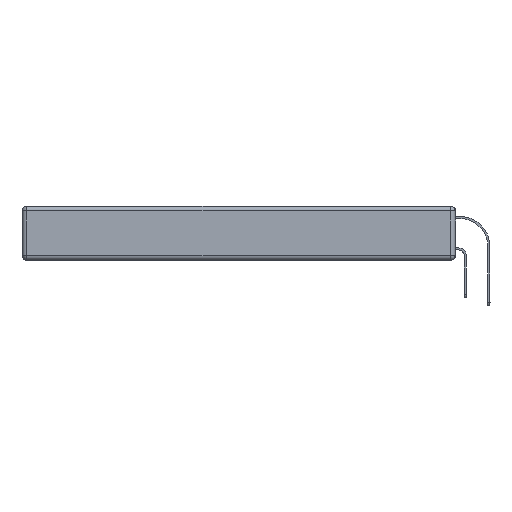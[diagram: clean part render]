
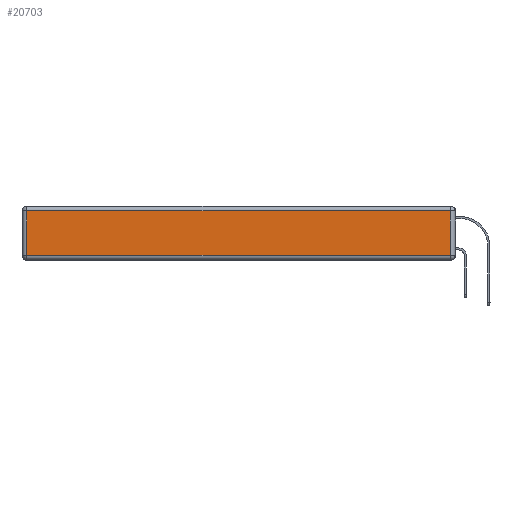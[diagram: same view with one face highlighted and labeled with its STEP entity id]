
A CAD part, left-side view. The second image highlights one B-rep face of the part: STEP entity #20703.
In plain terms, the highlighted planar face has unit normal (-1, 0, 0).
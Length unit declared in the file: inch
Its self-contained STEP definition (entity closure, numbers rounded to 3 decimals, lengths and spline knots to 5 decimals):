
#578 = VERTEX_POINT ( 'NONE', #16079 ) ;
#749 = EDGE_CURVE ( 'NONE', #12859, #14112, #18726, .T. ) ;
#1643 = VECTOR ( 'NONE', #2387, 39.37008 ) ;
#2387 = DIRECTION ( 'NONE',  ( 0., -1., 0. ) ) ;
#2833 = DIRECTION ( 'NONE',  ( 0., 0., 1. ) ) ;
#3191 = DIRECTION ( 'NONE',  ( 0., 0., 1. ) ) ;
#3199 = VERTEX_POINT ( 'NONE', #7223 ) ;
#3409 = VECTOR ( 'NONE', #21906, 39.37008 ) ;
#3702 = EDGE_CURVE ( 'NONE', #578, #3199, #10713, .T. ) ;
#4366 = ORIENTED_EDGE ( 'NONE', *, *, #13947, .T. ) ;
#4716 = EDGE_CURVE ( 'NONE', #3199, #12859, #5184, .T. ) ;
#5184 = LINE ( 'NONE', #16341, #3409 ) ;
#5561 = ORIENTED_EDGE ( 'NONE', *, *, #4716, .T. ) ;
#7223 = CARTESIAN_POINT ( 'NONE',  ( 0., 0.03, -0.03 ) ) ;
#7793 = ORIENTED_EDGE ( 'NONE', *, *, #749, .T. ) ;
#8169 = AXIS2_PLACEMENT_3D ( 'NONE', #17513, #13875, #2833 ) ;
#10346 = FACE_OUTER_BOUND ( 'NONE', #13433, .T. ) ;
#10713 = LINE ( 'NONE', #23314, #14962 ) ;
#11607 = LINE ( 'NONE', #19000, #1643 ) ;
#12859 = VERTEX_POINT ( 'NONE', #22223 ) ;
#13433 = EDGE_LOOP ( 'NONE', ( #4366, #23909, #5561, #7793 ) ) ;
#13875 = DIRECTION ( 'NONE',  ( -1., 0., 0. ) ) ;
#13947 = EDGE_CURVE ( 'NONE', #14112, #578, #11607, .T. ) ;
#14112 = VERTEX_POINT ( 'NONE', #21745 ) ;
#14962 = VECTOR ( 'NONE', #3191, 39.37008 ) ;
#16079 = CARTESIAN_POINT ( 'NONE',  ( 0., 0.03, -0.313 ) ) ;
#16341 = CARTESIAN_POINT ( 'NONE',  ( 0., 2.75, -0.03 ) ) ;
#17179 = VECTOR ( 'NONE', #22000, 39.37008 ) ;
#17513 = CARTESIAN_POINT ( 'NONE',  ( 0., 0., -0.343 ) ) ;
#18726 = LINE ( 'NONE', #20306, #17179 ) ;
#19000 = CARTESIAN_POINT ( 'NONE',  ( 0., 0., -0.313 ) ) ;
#20306 = CARTESIAN_POINT ( 'NONE',  ( 0., 2.72, -0.343 ) ) ;
#20703 = ADVANCED_FACE ( 'NONE', ( #10346 ), #21019, .T. ) ;
#21019 = PLANE ( 'NONE',  #8169 ) ;
#21745 = CARTESIAN_POINT ( 'NONE',  ( 0., 2.72, -0.313 ) ) ;
#21906 = DIRECTION ( 'NONE',  ( 0., 1., 0. ) ) ;
#22000 = DIRECTION ( 'NONE',  ( 0., 0., -1. ) ) ;
#22223 = CARTESIAN_POINT ( 'NONE',  ( 0., 2.72, -0.03 ) ) ;
#23314 = CARTESIAN_POINT ( 'NONE',  ( 0., 0.03, -0.343 ) ) ;
#23909 = ORIENTED_EDGE ( 'NONE', *, *, #3702, .T. ) ;
